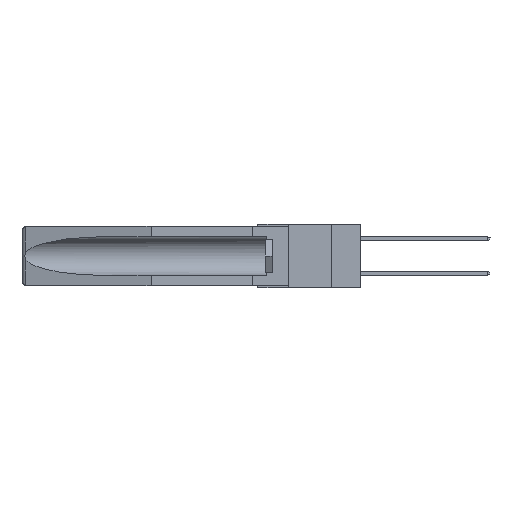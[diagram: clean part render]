
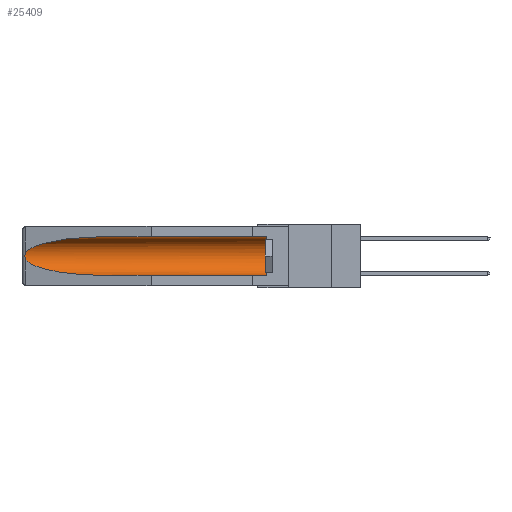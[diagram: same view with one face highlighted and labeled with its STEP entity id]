
A CAD part, left-side view. The second image highlights one B-rep face of the part: STEP entity #25409.
In plain terms, the highlighted cylindrical face has radius 2.857 mm (diameter 5.715 mm), a partial arc.
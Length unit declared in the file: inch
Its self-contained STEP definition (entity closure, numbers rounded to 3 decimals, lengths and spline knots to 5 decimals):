
#186 = EDGE_CURVE ( 'NONE', #23275, #12654, #18065, .T. ) ;
#446 = ORIENTED_EDGE ( 'NONE', *, *, #17488, .F. ) ;
#686 = DIRECTION ( 'NONE',  ( 0., 0., 1. ) ) ;
#1858 = VERTEX_POINT ( 'NONE', #13600 ) ;
#2373 = CARTESIAN_POINT ( 'NONE',  ( 0.26597, 1.52961, -0.15275 ) ) ;
#2636 = CARTESIAN_POINT ( 'NONE',  ( 0.155, -0.30754, -0.1715 ) ) ;
#2691 = DIRECTION ( 'NONE',  ( 0., -1., 0. ) ) ;
#4177 = EDGE_CURVE ( 'NONE', #14385, #23275, #17263, .T. ) ;
#4704 = CARTESIAN_POINT ( 'NONE',  ( 0.26537, 1.52718, -0.19328 ) ) ;
#4721 = CIRCLE ( 'NONE', #15282, 0.1125 ) ;
#4853 = CARTESIAN_POINT ( 'NONE',  ( 0.26537, 1.52718, -0.14972 ) ) ;
#4855 = CYLINDRICAL_SURFACE ( 'NONE', #11014, 0.1125 ) ;
#5598 = EDGE_CURVE ( 'NONE', #12654, #25265, #15388, .T. ) ;
#5886 = EDGE_CURVE ( 'NONE', #11457, #14385, #24858, .T. ) ;
#6130 = CARTESIAN_POINT ( 'NONE',  ( 0.26537, 1.52718, -0.19328 ) ) ;
#6615 = DIRECTION ( 'NONE',  ( 0., 0., 1. ) ) ;
#6647 = DIRECTION ( 'NONE',  ( 0., 1., 0. ) ) ;
#7141 = CARTESIAN_POINT ( 'NONE',  ( 0.155, -0.30754, -0.284 ) ) ;
#7178 = ORIENTED_EDGE ( 'NONE', *, *, #5886, .T. ) ;
#7436 = CARTESIAN_POINT ( 'NONE',  ( 0.155, -0.30754, -0.059 ) ) ;
#7523 = CARTESIAN_POINT ( 'NONE',  ( 0.21114, 1.30732, -0.059 ) ) ;
#8137 = CARTESIAN_POINT ( 'NONE',  ( 0.26597, 1.5296, -0.19026 ) ) ;
#8667 = ORIENTED_EDGE ( 'NONE', *, *, #186, .T. ) ;
#8856 = CARTESIAN_POINT ( 'NONE',  ( 0.2675, 1.53308, -0.16763 ) ) ;
#9250 = VECTOR ( 'NONE', #11059, 39.37008 ) ;
#9518 = CARTESIAN_POINT ( 'NONE',  ( 0.25451, 1.48313, -0.09465 ) ) ;
#10665 = CARTESIAN_POINT ( 'NONE',  ( 0.25451, 1.48313, -0.24835 ) ) ;
#10768 = ORIENTED_EDGE ( 'NONE', *, *, #4177, .T. ) ;
#11014 = AXIS2_PLACEMENT_3D ( 'NONE', #2636, #6647, #686 ) ;
#11059 = DIRECTION ( 'NONE',  ( 0., 1., 0. ) ) ;
#11353 = VECTOR ( 'NONE', #25323, 39.37008 ) ;
#11457 = VERTEX_POINT ( 'NONE', #16643 ) ;
#12654 = VERTEX_POINT ( 'NONE', #15117 ) ;
#12879 = CARTESIAN_POINT ( 'NONE',  ( 0.155, 0.126, -0.1715 ) ) ;
#12884 = CARTESIAN_POINT ( 'NONE',  ( 0.155, 1.07973, -0.284 ) ) ;
#13600 = CARTESIAN_POINT ( 'NONE',  ( 0.155, 0.126, -0.284 ) ) ;
#14385 = VERTEX_POINT ( 'NONE', #16770 ) ;
#14823 = CARTESIAN_POINT ( 'NONE',  ( 0.2675, 1.53308, -0.17534 ) ) ;
#15117 = CARTESIAN_POINT ( 'NONE',  ( 0.26537, 1.52718, -0.19328 ) ) ;
#15143 = LINE ( 'NONE', #7141, #9250 ) ;
#15282 = AXIS2_PLACEMENT_3D ( 'NONE', #12879, #2691, #6615 ) ;
#15388 =( BOUNDED_CURVE ( )  B_SPLINE_CURVE ( 3, ( #4704, #10665, #18624, #18453 ),
 .UNSPECIFIED., .F., .F. ) 
 B_SPLINE_CURVE_WITH_KNOTS ( ( 4, 4 ),
 ( 0.1948, 1.5708 ),
 .UNSPECIFIED. ) 
 CURVE ( )  GEOMETRIC_REPRESENTATION_ITEM ( )  RATIONAL_B_SPLINE_CURVE ( ( 1., 0.848, 0.848, 1. ) ) 
 REPRESENTATION_ITEM ( '' )  );
#16643 = CARTESIAN_POINT ( 'NONE',  ( 0.155, 0.126, -0.059 ) ) ;
#16770 = CARTESIAN_POINT ( 'NONE',  ( 0.155, 1.07973, -0.059 ) ) ;
#17263 =( BOUNDED_CURVE ( )  B_SPLINE_CURVE ( 3, ( #19354, #7523, #9518, #23287 ),
 .UNSPECIFIED., .F., .F. ) 
 B_SPLINE_CURVE_WITH_KNOTS ( ( 4, 4 ),
 ( 4.71239, 6.08839 ),
 .UNSPECIFIED. ) 
 CURVE ( )  GEOMETRIC_REPRESENTATION_ITEM ( )  RATIONAL_B_SPLINE_CURVE ( ( 1., 0.848, 0.848, 1. ) ) 
 REPRESENTATION_ITEM ( '' )  );
#17488 = EDGE_CURVE ( 'NONE', #1858, #25265, #15143, .T. ) ;
#18065 = B_SPLINE_CURVE_WITH_KNOTS ( 'NONE', 3,
 ( #4853, #2373, #23950, #18689, #8856, #14823, #24550, #21928, #8137, #6130 ),
 .UNSPECIFIED., .F., .F.,
 ( 4, 2, 2, 2, 4 ),
 ( 0., 0.00029, 0.00058, 0.00087, 0.00117 ),
 .UNSPECIFIED. ) ;
#18453 = CARTESIAN_POINT ( 'NONE',  ( 0.155, 1.07973, -0.284 ) ) ;
#18624 = CARTESIAN_POINT ( 'NONE',  ( 0.21114, 1.30732, -0.284 ) ) ;
#18689 = CARTESIAN_POINT ( 'NONE',  ( 0.2673, 1.5327, -0.16383 ) ) ;
#19354 = CARTESIAN_POINT ( 'NONE',  ( 0.155, 1.07973, -0.059 ) ) ;
#20660 = EDGE_CURVE ( 'NONE', #1858, #11457, #4721, .T. ) ;
#21506 = FACE_OUTER_BOUND ( 'NONE', #22703, .T. ) ;
#21928 = CARTESIAN_POINT ( 'NONE',  ( 0.26655, 1.53094, -0.18657 ) ) ;
#22250 = ORIENTED_EDGE ( 'NONE', *, *, #20660, .T. ) ;
#22703 = EDGE_LOOP ( 'NONE', ( #10768, #8667, #24934, #446, #22250, #7178 ) ) ;
#23275 = VERTEX_POINT ( 'NONE', #24204 ) ;
#23287 = CARTESIAN_POINT ( 'NONE',  ( 0.26537, 1.52718, -0.14972 ) ) ;
#23950 = CARTESIAN_POINT ( 'NONE',  ( 0.26654, 1.53092, -0.15636 ) ) ;
#24204 = CARTESIAN_POINT ( 'NONE',  ( 0.26537, 1.52718, -0.14972 ) ) ;
#24550 = CARTESIAN_POINT ( 'NONE',  ( 0.2673, 1.53269, -0.17917 ) ) ;
#24858 = LINE ( 'NONE', #7436, #11353 ) ;
#24934 = ORIENTED_EDGE ( 'NONE', *, *, #5598, .T. ) ;
#25265 = VERTEX_POINT ( 'NONE', #12884 ) ;
#25323 = DIRECTION ( 'NONE',  ( 0., 1., 0. ) ) ;
#25409 = ADVANCED_FACE ( 'NONE', ( #21506 ), #4855, .F. ) ;
